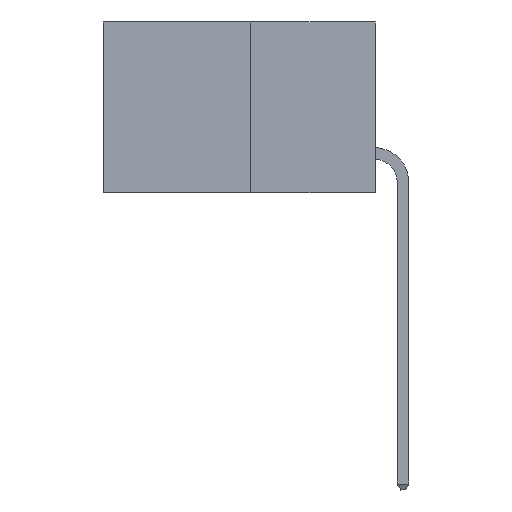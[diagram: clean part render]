
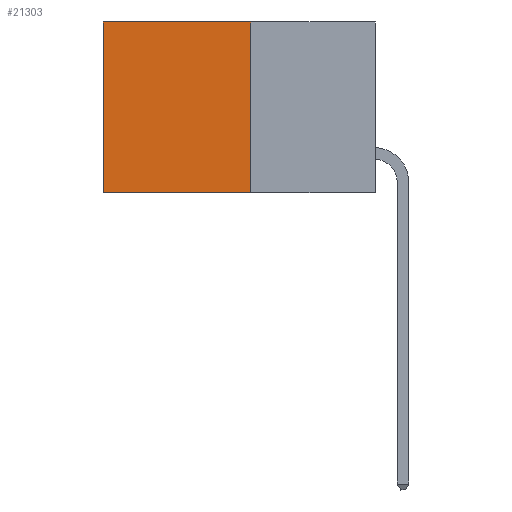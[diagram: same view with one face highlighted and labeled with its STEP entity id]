
A CAD part, left-side view. The second image highlights one B-rep face of the part: STEP entity #21303.
In plain terms, the highlighted planar face has unit normal (-1, 0, 0).
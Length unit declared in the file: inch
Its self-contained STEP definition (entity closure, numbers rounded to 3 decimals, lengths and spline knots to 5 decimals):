
#711 = DIRECTION ( 'NONE',  ( 0., 1., 0. ) ) ;
#3010 = VECTOR ( 'NONE', #27981, 39.37008 ) ;
#3888 = CARTESIAN_POINT ( 'NONE',  ( 0.277, 0.27, -0.37 ) ) ;
#5482 = VERTEX_POINT ( 'NONE', #29643 ) ;
#5682 = CARTESIAN_POINT ( 'NONE',  ( 0.277, 0.59, -0.37 ) ) ;
#6293 = VECTOR ( 'NONE', #8143, 39.37008 ) ;
#6407 = DIRECTION ( 'NONE',  ( 0., 0., -1. ) ) ;
#6543 = FACE_OUTER_BOUND ( 'NONE', #9314, .T. ) ;
#6661 = CARTESIAN_POINT ( 'NONE',  ( 0.277, 0.59, 0. ) ) ;
#7435 = DIRECTION ( 'NONE',  ( 0., 1., 0. ) ) ;
#8143 = DIRECTION ( 'NONE',  ( 0., 0., -1. ) ) ;
#9314 = EDGE_LOOP ( 'NONE', ( #15289, #26102, #15701, #19848 ) ) ;
#9867 = CARTESIAN_POINT ( 'NONE',  ( 0.277, 0.27, -0.37 ) ) ;
#10467 = LINE ( 'NONE', #5682, #3010 ) ;
#11114 = EDGE_CURVE ( 'NONE', #5482, #25540, #21053, .T. ) ;
#13228 = EDGE_CURVE ( 'NONE', #25540, #22100, #10467, .T. ) ;
#13431 = CARTESIAN_POINT ( 'NONE',  ( 0.277, 0.27, -0.37 ) ) ;
#14440 = VECTOR ( 'NONE', #711, 39.37008 ) ;
#15289 = ORIENTED_EDGE ( 'NONE', *, *, #13228, .T. ) ;
#15701 = ORIENTED_EDGE ( 'NONE', *, *, #24534, .F. ) ;
#16340 = PLANE ( 'NONE',  #30887 ) ;
#16722 = CARTESIAN_POINT ( 'NONE',  ( 0.277, 0.59, -0.37 ) ) ;
#16893 = EDGE_CURVE ( 'NONE', #25363, #22100, #31168, .T. ) ;
#19848 = ORIENTED_EDGE ( 'NONE', *, *, #11114, .T. ) ;
#20316 = LINE ( 'NONE', #30258, #6293 ) ;
#21053 = LINE ( 'NONE', #22919, #14440 ) ;
#21303 = ADVANCED_FACE ( 'NONE', ( #6543 ), #16340, .F. ) ;
#21310 = DIRECTION ( 'NONE',  ( 1., 0., 0. ) ) ;
#22100 = VERTEX_POINT ( 'NONE', #16722 ) ;
#22919 = CARTESIAN_POINT ( 'NONE',  ( 0.277, 0.27, 0. ) ) ;
#24534 = EDGE_CURVE ( 'NONE', #5482, #25363, #20316, .T. ) ;
#24614 = VECTOR ( 'NONE', #7435, 39.37008 ) ;
#25363 = VERTEX_POINT ( 'NONE', #13431 ) ;
#25540 = VERTEX_POINT ( 'NONE', #6661 ) ;
#26102 = ORIENTED_EDGE ( 'NONE', *, *, #16893, .F. ) ;
#27981 = DIRECTION ( 'NONE',  ( 0., 0., -1. ) ) ;
#29643 = CARTESIAN_POINT ( 'NONE',  ( 0.277, 0.27, 0. ) ) ;
#30258 = CARTESIAN_POINT ( 'NONE',  ( 0.277, 0.27, -0.37 ) ) ;
#30887 = AXIS2_PLACEMENT_3D ( 'NONE', #3888, #21310, #6407 ) ;
#31168 = LINE ( 'NONE', #9867, #24614 ) ;
